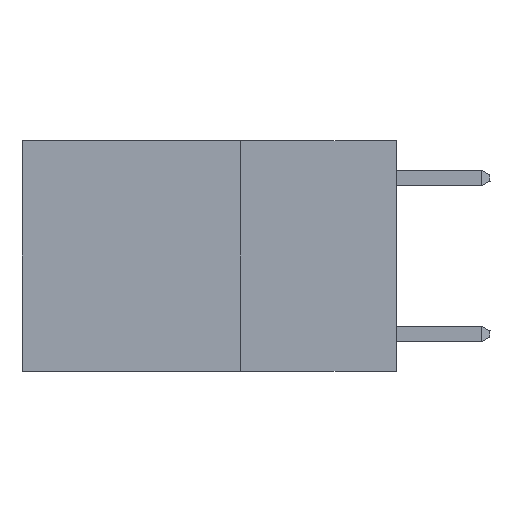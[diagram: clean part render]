
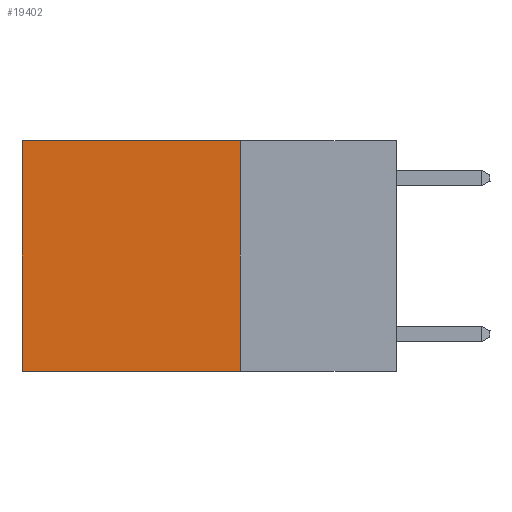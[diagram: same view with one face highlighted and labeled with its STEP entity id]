
A CAD part, left-side view. The second image highlights one B-rep face of the part: STEP entity #19402.
In plain terms, the highlighted planar face has unit normal (-1, 0, 0).
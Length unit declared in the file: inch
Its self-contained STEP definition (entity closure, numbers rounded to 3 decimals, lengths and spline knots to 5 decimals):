
#1430 = VERTEX_POINT ( 'NONE', #11859 ) ;
#1718 = FACE_OUTER_BOUND ( 'NONE', #3254, .T. ) ;
#2243 = CARTESIAN_POINT ( 'NONE',  ( 0.2625, 0.25, 0. ) ) ;
#3254 = EDGE_LOOP ( 'NONE', ( #24555, #25501, #28916, #17147 ) ) ;
#4503 = DIRECTION ( 'NONE',  ( 0., 0., -1. ) ) ;
#4978 = LINE ( 'NONE', #31457, #23881 ) ;
#8836 = LINE ( 'NONE', #14299, #20316 ) ;
#9743 = DIRECTION ( 'NONE',  ( 0., 1., 0. ) ) ;
#11079 = VERTEX_POINT ( 'NONE', #14085 ) ;
#11082 = CARTESIAN_POINT ( 'NONE',  ( 0.2625, 0.6, 0. ) ) ;
#11623 = VERTEX_POINT ( 'NONE', #16205 ) ;
#11859 = CARTESIAN_POINT ( 'NONE',  ( 0.2625, 0.6, -0.37 ) ) ;
#12165 = DIRECTION ( 'NONE',  ( 0., 1., 0. ) ) ;
#12339 = AXIS2_PLACEMENT_3D ( 'NONE', #19415, #29147, #14636 ) ;
#12772 = EDGE_CURVE ( 'NONE', #24992, #1430, #8836, .T. ) ;
#14085 = CARTESIAN_POINT ( 'NONE',  ( 0.2625, 0.25, -0.37 ) ) ;
#14299 = CARTESIAN_POINT ( 'NONE',  ( 0.2625, 0.6, 0. ) ) ;
#14636 = DIRECTION ( 'NONE',  ( 0., 0., -1. ) ) ;
#15351 = EDGE_CURVE ( 'NONE', #11623, #24992, #18591, .T. ) ;
#16205 = CARTESIAN_POINT ( 'NONE',  ( 0.2625, 0.25, 0. ) ) ;
#16369 = EDGE_CURVE ( 'NONE', #11623, #11079, #24197, .T. ) ;
#17147 = ORIENTED_EDGE ( 'NONE', *, *, #15351, .T. ) ;
#17757 = VECTOR ( 'NONE', #18268, 39.37008 ) ;
#18268 = DIRECTION ( 'NONE',  ( 0., 0., -1. ) ) ;
#18591 = LINE ( 'NONE', #2243, #30654 ) ;
#19402 = ADVANCED_FACE ( 'NONE', ( #1718 ), #24262, .F. ) ;
#19406 = EDGE_CURVE ( 'NONE', #11079, #1430, #4978, .T. ) ;
#19415 = CARTESIAN_POINT ( 'NONE',  ( 0.2625, 0.25, 0. ) ) ;
#20316 = VECTOR ( 'NONE', #4503, 39.37008 ) ;
#23242 = CARTESIAN_POINT ( 'NONE',  ( 0.2625, 0.25, 0. ) ) ;
#23881 = VECTOR ( 'NONE', #12165, 39.37008 ) ;
#24197 = LINE ( 'NONE', #23242, #17757 ) ;
#24262 = PLANE ( 'NONE',  #12339 ) ;
#24555 = ORIENTED_EDGE ( 'NONE', *, *, #12772, .T. ) ;
#24992 = VERTEX_POINT ( 'NONE', #11082 ) ;
#25501 = ORIENTED_EDGE ( 'NONE', *, *, #19406, .F. ) ;
#28916 = ORIENTED_EDGE ( 'NONE', *, *, #16369, .F. ) ;
#29147 = DIRECTION ( 'NONE',  ( 1., 0., 0. ) ) ;
#30654 = VECTOR ( 'NONE', #9743, 39.37008 ) ;
#31457 = CARTESIAN_POINT ( 'NONE',  ( 0.2625, 0.25, -0.37 ) ) ;
